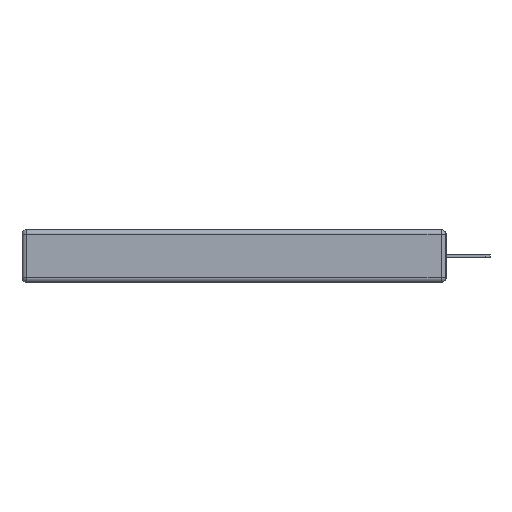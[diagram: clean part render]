
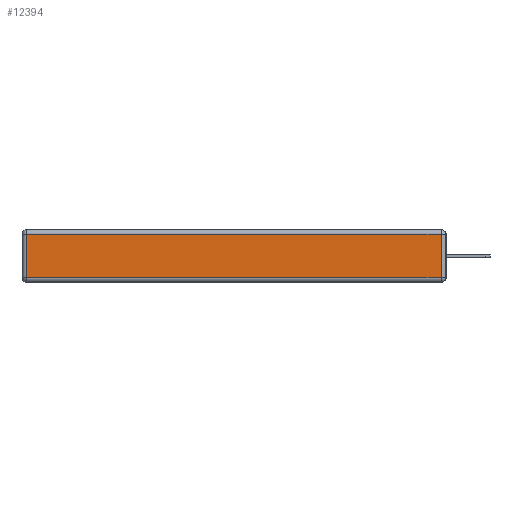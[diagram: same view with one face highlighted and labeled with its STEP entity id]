
A CAD part, left-side view. The second image highlights one B-rep face of the part: STEP entity #12394.
In plain terms, the highlighted planar face has unit normal (-1, 0, 0).
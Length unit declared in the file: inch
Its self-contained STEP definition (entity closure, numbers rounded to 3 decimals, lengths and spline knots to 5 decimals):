
#145 = CARTESIAN_POINT ( 'NONE',  ( 0., 2.75, -0.03 ) ) ;
#959 = LINE ( 'NONE', #11059, #6627 ) ;
#1241 = CARTESIAN_POINT ( 'NONE',  ( 0., 0., -0.343 ) ) ;
#1496 = VECTOR ( 'NONE', #7131, 39.37008 ) ;
#2066 = CARTESIAN_POINT ( 'NONE',  ( 0., 2.72, -0.03 ) ) ;
#2122 = AXIS2_PLACEMENT_3D ( 'NONE', #1241, #3637, #11089 ) ;
#2239 = LINE ( 'NONE', #6062, #1496 ) ;
#2441 = PLANE ( 'NONE',  #2122 ) ;
#2488 = DIRECTION ( 'NONE',  ( 0., 1., 0. ) ) ;
#2682 = LINE ( 'NONE', #12036, #10938 ) ;
#3587 = ORIENTED_EDGE ( 'NONE', *, *, #8853, .T. ) ;
#3630 = ORIENTED_EDGE ( 'NONE', *, *, #9544, .T. ) ;
#3637 = DIRECTION ( 'NONE',  ( -1., 0., 0. ) ) ;
#3714 = CARTESIAN_POINT ( 'NONE',  ( 0., 0.03, -0.313 ) ) ;
#4702 = DIRECTION ( 'NONE',  ( 0., 0., 1. ) ) ;
#4747 = ORIENTED_EDGE ( 'NONE', *, *, #13710, .T. ) ;
#4821 = DIRECTION ( 'NONE',  ( 0., 0., -1. ) ) ;
#5203 = EDGE_LOOP ( 'NONE', ( #4747, #11890, #3630, #3587 ) ) ;
#6062 = CARTESIAN_POINT ( 'NONE',  ( 0., 0., -0.313 ) ) ;
#6446 = LINE ( 'NONE', #145, #11688 ) ;
#6611 = CARTESIAN_POINT ( 'NONE',  ( 0., 0.03, -0.03 ) ) ;
#6627 = VECTOR ( 'NONE', #4821, 39.37008 ) ;
#7131 = DIRECTION ( 'NONE',  ( 0., -1., 0. ) ) ;
#8853 = EDGE_CURVE ( 'NONE', #13515, #13166, #959, .T. ) ;
#9544 = EDGE_CURVE ( 'NONE', #10629, #13515, #6446, .T. ) ;
#10215 = VERTEX_POINT ( 'NONE', #3714 ) ;
#10629 = VERTEX_POINT ( 'NONE', #6611 ) ;
#10938 = VECTOR ( 'NONE', #4702, 39.37008 ) ;
#11059 = CARTESIAN_POINT ( 'NONE',  ( 0., 2.72, -0.343 ) ) ;
#11089 = DIRECTION ( 'NONE',  ( 0., 0., 1. ) ) ;
#11688 = VECTOR ( 'NONE', #2488, 39.37008 ) ;
#11890 = ORIENTED_EDGE ( 'NONE', *, *, #12340, .T. ) ;
#12036 = CARTESIAN_POINT ( 'NONE',  ( 0., 0.03, -0.343 ) ) ;
#12340 = EDGE_CURVE ( 'NONE', #10215, #10629, #2682, .T. ) ;
#12394 = ADVANCED_FACE ( 'NONE', ( #13669 ), #2441, .T. ) ;
#13166 = VERTEX_POINT ( 'NONE', #13328 ) ;
#13328 = CARTESIAN_POINT ( 'NONE',  ( 0., 2.72, -0.313 ) ) ;
#13515 = VERTEX_POINT ( 'NONE', #2066 ) ;
#13669 = FACE_OUTER_BOUND ( 'NONE', #5203, .T. ) ;
#13710 = EDGE_CURVE ( 'NONE', #13166, #10215, #2239, .T. ) ;
